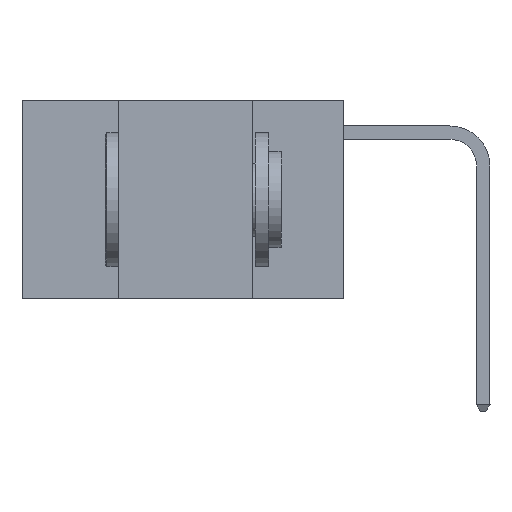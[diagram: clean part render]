
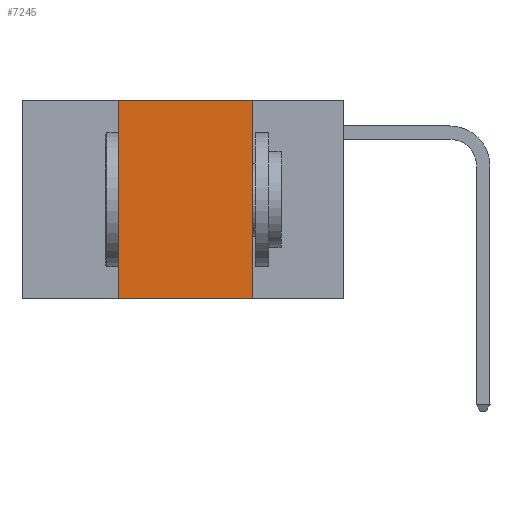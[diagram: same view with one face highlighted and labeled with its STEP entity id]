
A CAD part, left-side view. The second image highlights one B-rep face of the part: STEP entity #7245.
In plain terms, the highlighted planar face has unit normal (-1, 0, 0).
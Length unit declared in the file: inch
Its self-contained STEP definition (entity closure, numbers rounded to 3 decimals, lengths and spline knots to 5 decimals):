
#776 = ORIENTED_EDGE ( 'NONE', *, *, #7166, .T. ) ;
#843 = EDGE_LOOP ( 'NONE', ( #17901, #23675, #13527, #776 ) ) ;
#1267 = FACE_OUTER_BOUND ( 'NONE', #843, .T. ) ;
#1358 = CARTESIAN_POINT ( 'NONE',  ( 0., 0.6, -0.37 ) ) ;
#3657 = DIRECTION ( 'NONE',  ( 0., 0., -1. ) ) ;
#3815 = LINE ( 'NONE', #1358, #18250 ) ;
#4896 = VECTOR ( 'NONE', #6723, 39.37008 ) ;
#4925 = CARTESIAN_POINT ( 'NONE',  ( 0., 0.6, 0. ) ) ;
#6213 = CARTESIAN_POINT ( 'NONE',  ( 0., 0.42, 0. ) ) ;
#6488 = CARTESIAN_POINT ( 'NONE',  ( 0., 0.17, 0. ) ) ;
#6723 = DIRECTION ( 'NONE',  ( 0., -1., 0. ) ) ;
#7166 = EDGE_CURVE ( 'NONE', #7426, #10806, #3815, .T. ) ;
#7245 = ADVANCED_FACE ( 'NONE', ( #1267 ), #13449, .F. ) ;
#7426 = VERTEX_POINT ( 'NONE', #15918 ) ;
#8102 = VERTEX_POINT ( 'NONE', #6488 ) ;
#10091 = VECTOR ( 'NONE', #18502, 39.37008 ) ;
#10106 = AXIS2_PLACEMENT_3D ( 'NONE', #23198, #15412, #3657 ) ;
#10717 = LINE ( 'NONE', #18417, #10091 ) ;
#10800 = CARTESIAN_POINT ( 'NONE',  ( 0., 0.17, -0.37 ) ) ;
#10806 = VERTEX_POINT ( 'NONE', #10800 ) ;
#11217 = DIRECTION ( 'NONE',  ( 0., -1., 0. ) ) ;
#12385 = VECTOR ( 'NONE', #21866, 39.37008 ) ;
#13449 = PLANE ( 'NONE',  #10106 ) ;
#13527 = ORIENTED_EDGE ( 'NONE', *, *, #13707, .F. ) ;
#13707 = EDGE_CURVE ( 'NONE', #7426, #17318, #22166, .T. ) ;
#15412 = DIRECTION ( 'NONE',  ( 1., 0., 0. ) ) ;
#15918 = CARTESIAN_POINT ( 'NONE',  ( 0., 0.42, -0.37 ) ) ;
#16084 = CARTESIAN_POINT ( 'NONE',  ( 0., 0.42, 0. ) ) ;
#16229 = EDGE_CURVE ( 'NONE', #17318, #8102, #20503, .T. ) ;
#17318 = VERTEX_POINT ( 'NONE', #16084 ) ;
#17901 = ORIENTED_EDGE ( 'NONE', *, *, #18977, .F. ) ;
#18250 = VECTOR ( 'NONE', #11217, 39.37008 ) ;
#18417 = CARTESIAN_POINT ( 'NONE',  ( 0., 0.17, 0. ) ) ;
#18502 = DIRECTION ( 'NONE',  ( 0., 0., -1. ) ) ;
#18977 = EDGE_CURVE ( 'NONE', #8102, #10806, #10717, .T. ) ;
#20503 = LINE ( 'NONE', #4925, #4896 ) ;
#21866 = DIRECTION ( 'NONE',  ( 0., 0., 1. ) ) ;
#22166 = LINE ( 'NONE', #6213, #12385 ) ;
#23198 = CARTESIAN_POINT ( 'NONE',  ( 0., 0.6, 0. ) ) ;
#23675 = ORIENTED_EDGE ( 'NONE', *, *, #16229, .F. ) ;
